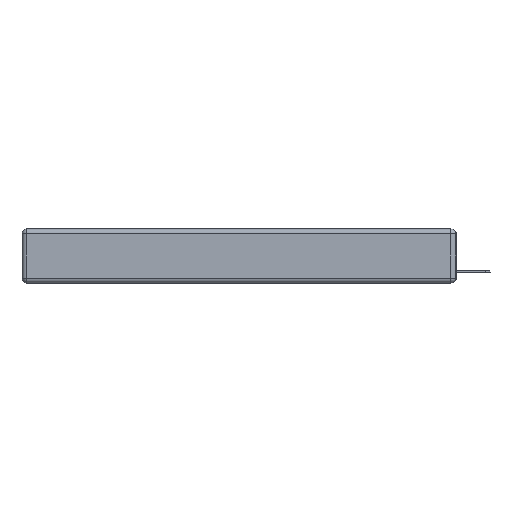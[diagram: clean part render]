
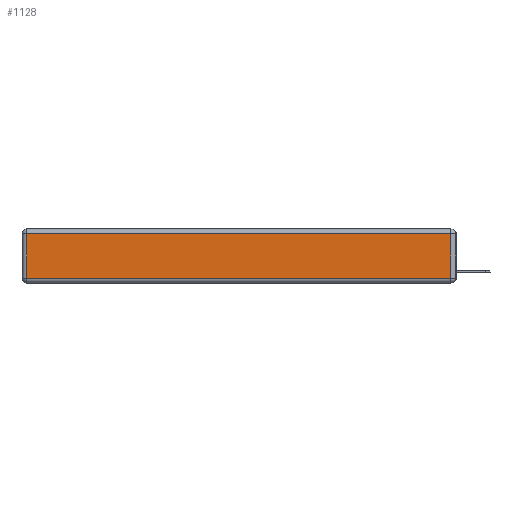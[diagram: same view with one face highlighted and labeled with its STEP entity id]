
A CAD part, left-side view. The second image highlights one B-rep face of the part: STEP entity #1128.
In plain terms, the highlighted planar face has unit normal (-1, 0, 0).
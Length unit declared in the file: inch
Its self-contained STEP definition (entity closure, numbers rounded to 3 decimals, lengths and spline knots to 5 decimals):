
#5 = CARTESIAN_POINT ( 'NONE',  ( 0., 0.03, -0.313 ) ) ;
#507 = LINE ( 'NONE', #13292, #4966 ) ;
#1128 = ADVANCED_FACE ( 'NONE', ( #6149 ), #9256, .T. ) ;
#1211 = EDGE_CURVE ( 'NONE', #6784, #3504, #2352, .T. ) ;
#1500 = AXIS2_PLACEMENT_3D ( 'NONE', #10506, #13523, #3913 ) ;
#1570 = DIRECTION ( 'NONE',  ( 0., 1., 0. ) ) ;
#2286 = EDGE_CURVE ( 'NONE', #5179, #5635, #4801, .T. ) ;
#2314 = CARTESIAN_POINT ( 'NONE',  ( 0., 0.03, -0.03 ) ) ;
#2345 = ORIENTED_EDGE ( 'NONE', *, *, #3578, .T. ) ;
#2352 = LINE ( 'NONE', #4326, #9089 ) ;
#2695 = CARTESIAN_POINT ( 'NONE',  ( 0., 0.03, -0.343 ) ) ;
#3504 = VERTEX_POINT ( 'NONE', #3743 ) ;
#3578 = EDGE_CURVE ( 'NONE', #5635, #6784, #507, .T. ) ;
#3743 = CARTESIAN_POINT ( 'NONE',  ( 0., 2.72, -0.313 ) ) ;
#3913 = DIRECTION ( 'NONE',  ( 0., 0., 1. ) ) ;
#4154 = DIRECTION ( 'NONE',  ( 0., -1., 0. ) ) ;
#4326 = CARTESIAN_POINT ( 'NONE',  ( 0., 2.72, -0.343 ) ) ;
#4801 = LINE ( 'NONE', #2695, #7166 ) ;
#4966 = VECTOR ( 'NONE', #1570, 39.37008 ) ;
#5072 = ORIENTED_EDGE ( 'NONE', *, *, #2286, .T. ) ;
#5179 = VERTEX_POINT ( 'NONE', #5 ) ;
#5512 = EDGE_LOOP ( 'NONE', ( #7606, #5072, #2345, #13045 ) ) ;
#5635 = VERTEX_POINT ( 'NONE', #2314 ) ;
#5799 = CARTESIAN_POINT ( 'NONE',  ( 0., 2.72, -0.03 ) ) ;
#6149 = FACE_OUTER_BOUND ( 'NONE', #5512, .T. ) ;
#6784 = VERTEX_POINT ( 'NONE', #5799 ) ;
#7166 = VECTOR ( 'NONE', #8862, 39.37008 ) ;
#7606 = ORIENTED_EDGE ( 'NONE', *, *, #13450, .T. ) ;
#8862 = DIRECTION ( 'NONE',  ( 0., 0., 1. ) ) ;
#9089 = VECTOR ( 'NONE', #11843, 39.37008 ) ;
#9256 = PLANE ( 'NONE',  #1500 ) ;
#9496 = LINE ( 'NONE', #13766, #10593 ) ;
#10506 = CARTESIAN_POINT ( 'NONE',  ( 0., 0., -0.343 ) ) ;
#10593 = VECTOR ( 'NONE', #4154, 39.37008 ) ;
#11843 = DIRECTION ( 'NONE',  ( 0., 0., -1. ) ) ;
#13045 = ORIENTED_EDGE ( 'NONE', *, *, #1211, .T. ) ;
#13292 = CARTESIAN_POINT ( 'NONE',  ( 0., 2.75, -0.03 ) ) ;
#13450 = EDGE_CURVE ( 'NONE', #3504, #5179, #9496, .T. ) ;
#13523 = DIRECTION ( 'NONE',  ( -1., 0., 0. ) ) ;
#13766 = CARTESIAN_POINT ( 'NONE',  ( 0., 0., -0.313 ) ) ;
